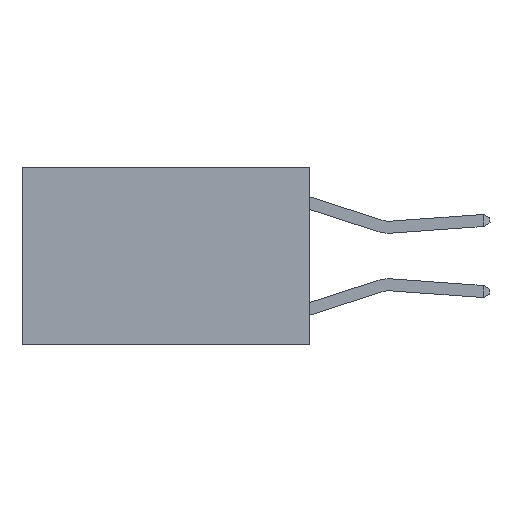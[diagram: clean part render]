
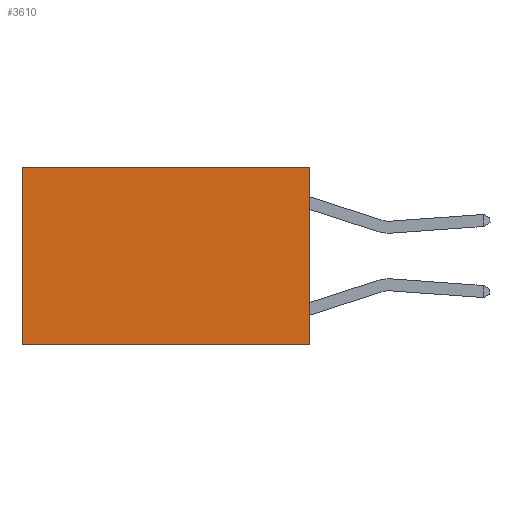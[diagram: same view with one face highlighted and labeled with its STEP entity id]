
A CAD part, left-side view. The second image highlights one B-rep face of the part: STEP entity #3610.
In plain terms, the highlighted planar face has unit normal (-1, 0, 0).
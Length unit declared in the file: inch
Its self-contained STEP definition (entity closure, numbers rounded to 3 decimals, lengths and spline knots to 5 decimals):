
#85 = EDGE_LOOP ( 'NONE', ( #676, #9103, #11006, #8152 ) ) ;
#272 = DIRECTION ( 'NONE',  ( 0., 1., 0. ) ) ;
#311 = VECTOR ( 'NONE', #272, 39.37008 ) ;
#676 = ORIENTED_EDGE ( 'NONE', *, *, #3295, .T. ) ;
#704 = CARTESIAN_POINT ( 'NONE',  ( 0.2625, 0., 0. ) ) ;
#863 = LINE ( 'NONE', #2539, #10732 ) ;
#1564 = VECTOR ( 'NONE', #7647, 39.37008 ) ;
#1608 = EDGE_CURVE ( 'NONE', #7654, #9716, #2898, .T. ) ;
#2163 = VERTEX_POINT ( 'NONE', #8941 ) ;
#2539 = CARTESIAN_POINT ( 'NONE',  ( 0.2625, 0.6, 0. ) ) ;
#2898 = LINE ( 'NONE', #5466, #311 ) ;
#3255 = VECTOR ( 'NONE', #7732, 39.37008 ) ;
#3295 = EDGE_CURVE ( 'NONE', #2163, #9716, #863, .T. ) ;
#3454 = CARTESIAN_POINT ( 'NONE',  ( 0.2625, 0., 0. ) ) ;
#3540 = LINE ( 'NONE', #3454, #3255 ) ;
#3610 = ADVANCED_FACE ( 'NONE', ( #6409 ), #3656, .F. ) ;
#3656 = PLANE ( 'NONE',  #5554 ) ;
#4875 = EDGE_CURVE ( 'NONE', #9958, #2163, #3540, .T. ) ;
#5109 = CARTESIAN_POINT ( 'NONE',  ( 0.2625, 0., -0.37 ) ) ;
#5466 = CARTESIAN_POINT ( 'NONE',  ( 0.2625, 0., -0.37 ) ) ;
#5554 = AXIS2_PLACEMENT_3D ( 'NONE', #7260, #6482, #10818 ) ;
#6409 = FACE_OUTER_BOUND ( 'NONE', #85, .T. ) ;
#6482 = DIRECTION ( 'NONE',  ( 1., 0., 0. ) ) ;
#7136 = LINE ( 'NONE', #704, #1564 ) ;
#7226 = EDGE_CURVE ( 'NONE', #9958, #7654, #7136, .T. ) ;
#7260 = CARTESIAN_POINT ( 'NONE',  ( 0.2625, 0., 0. ) ) ;
#7647 = DIRECTION ( 'NONE',  ( 0., 0., -1. ) ) ;
#7654 = VERTEX_POINT ( 'NONE', #5109 ) ;
#7732 = DIRECTION ( 'NONE',  ( 0., 1., 0. ) ) ;
#7800 = DIRECTION ( 'NONE',  ( 0., 0., -1. ) ) ;
#8152 = ORIENTED_EDGE ( 'NONE', *, *, #4875, .T. ) ;
#8366 = CARTESIAN_POINT ( 'NONE',  ( 0.2625, 0.6, -0.37 ) ) ;
#8941 = CARTESIAN_POINT ( 'NONE',  ( 0.2625, 0.6, 0. ) ) ;
#9103 = ORIENTED_EDGE ( 'NONE', *, *, #1608, .F. ) ;
#9716 = VERTEX_POINT ( 'NONE', #8366 ) ;
#9827 = CARTESIAN_POINT ( 'NONE',  ( 0.2625, 0., 0. ) ) ;
#9958 = VERTEX_POINT ( 'NONE', #9827 ) ;
#10732 = VECTOR ( 'NONE', #7800, 39.37008 ) ;
#10818 = DIRECTION ( 'NONE',  ( 0., 0., -1. ) ) ;
#11006 = ORIENTED_EDGE ( 'NONE', *, *, #7226, .F. ) ;
